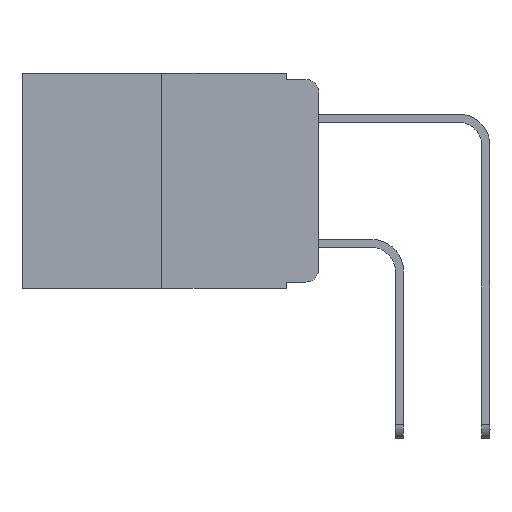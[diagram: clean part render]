
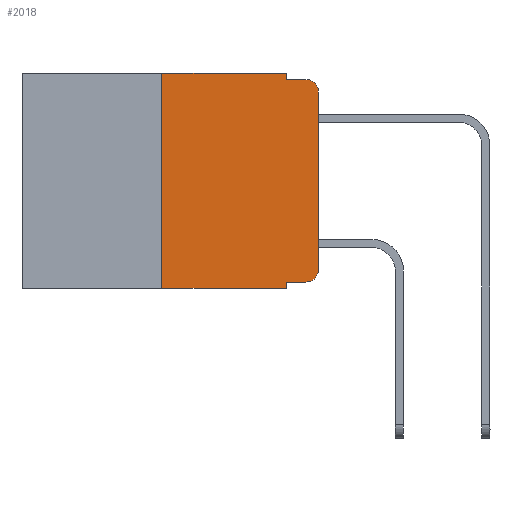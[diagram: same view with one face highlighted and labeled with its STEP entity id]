
A CAD part, left-side view. The second image highlights one B-rep face of the part: STEP entity #2018.
In plain terms, the highlighted planar face has unit normal (-1, 0, 0).
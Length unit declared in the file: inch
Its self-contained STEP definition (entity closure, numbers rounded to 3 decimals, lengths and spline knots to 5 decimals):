
#422 = EDGE_CURVE ( 'NONE', #14322, #1639, #7093, .T. ) ;
#611 = CARTESIAN_POINT ( 'NONE',  ( 0., 0.25, 0. ) ) ;
#840 = CARTESIAN_POINT ( 'NONE',  ( 0., 0.051, -0.333 ) ) ;
#1076 = EDGE_LOOP ( 'NONE', ( #9574, #23287, #19978, #2584, #23027, #23649, #20251, #6102, #7151, #8099 ) ) ;
#1297 = CARTESIAN_POINT ( 'NONE',  ( 0., 0.25, 0. ) ) ;
#1639 = VERTEX_POINT ( 'NONE', #19466 ) ;
#2018 = ADVANCED_FACE ( 'NONE', ( #4429 ), #2615, .F. ) ;
#2118 = CARTESIAN_POINT ( 'NONE',  ( 0., 0.051, 0. ) ) ;
#2147 = VERTEX_POINT ( 'NONE', #840 ) ;
#2360 = CARTESIAN_POINT ( 'NONE',  ( 0., 0.02, -0.03 ) ) ;
#2584 = ORIENTED_EDGE ( 'NONE', *, *, #422, .F. ) ;
#2593 = DIRECTION ( 'NONE',  ( 0., -1., 0. ) ) ;
#2615 = PLANE ( 'NONE',  #22516 ) ;
#2721 = DIRECTION ( 'NONE',  ( 0., 0., -1. ) ) ;
#2748 = VECTOR ( 'NONE', #12771, 39.37008 ) ;
#2932 = VECTOR ( 'NONE', #7549, 39.37008 ) ;
#3900 = DIRECTION ( 'NONE',  ( 0., -1., 0. ) ) ;
#3923 = EDGE_CURVE ( 'NONE', #11916, #7514, #4815, .T. ) ;
#4429 = FACE_OUTER_BOUND ( 'NONE', #1076, .T. ) ;
#4815 = LINE ( 'NONE', #10247, #19040 ) ;
#4859 = VECTOR ( 'NONE', #5276, 39.37008 ) ;
#4883 = VECTOR ( 'NONE', #5270, 39.37008 ) ;
#5023 = EDGE_CURVE ( 'NONE', #5339, #14322, #12719, .T. ) ;
#5270 = DIRECTION ( 'NONE',  ( 0., 0., 1. ) ) ;
#5276 = DIRECTION ( 'NONE',  ( 0., 0., 1. ) ) ;
#5339 = VERTEX_POINT ( 'NONE', #611 ) ;
#5505 = CARTESIAN_POINT ( 'NONE',  ( 0., 0.051, -0.343 ) ) ;
#6102 = ORIENTED_EDGE ( 'NONE', *, *, #18619, .F. ) ;
#6596 = DIRECTION ( 'NONE',  ( 1., 0., 0. ) ) ;
#6628 = EDGE_CURVE ( 'NONE', #2147, #13304, #19169, .T. ) ;
#7093 = LINE ( 'NONE', #19825, #2748 ) ;
#7151 = ORIENTED_EDGE ( 'NONE', *, *, #6628, .T. ) ;
#7514 = VERTEX_POINT ( 'NONE', #5505 ) ;
#7549 = DIRECTION ( 'NONE',  ( 0., 0., -1. ) ) ;
#8099 = ORIENTED_EDGE ( 'NONE', *, *, #9639, .T. ) ;
#8735 = CIRCLE ( 'NONE', #19583, 0.02 ) ;
#9193 = DIRECTION ( 'NONE',  ( 0., 0., -1. ) ) ;
#9363 = LINE ( 'NONE', #2118, #2932 ) ;
#9413 = VERTEX_POINT ( 'NONE', #15880 ) ;
#9574 = ORIENTED_EDGE ( 'NONE', *, *, #19260, .T. ) ;
#9639 = EDGE_CURVE ( 'NONE', #13304, #9413, #15652, .T. ) ;
#9912 = VECTOR ( 'NONE', #10658, 39.37008 ) ;
#9978 = CARTESIAN_POINT ( 'NONE',  ( 0., 0.473, 0. ) ) ;
#10247 = CARTESIAN_POINT ( 'NONE',  ( 0., 0.473, -0.343 ) ) ;
#10317 = VECTOR ( 'NONE', #2593, 39.37008 ) ;
#10330 = CARTESIAN_POINT ( 'NONE',  ( 0., 0.051, -0.333 ) ) ;
#10658 = DIRECTION ( 'NONE',  ( 0., -1., 0. ) ) ;
#11916 = VERTEX_POINT ( 'NONE', #13614 ) ;
#12398 = VERTEX_POINT ( 'NONE', #16133 ) ;
#12719 = LINE ( 'NONE', #23633, #9912 ) ;
#12734 = EDGE_CURVE ( 'NONE', #1639, #22343, #19135, .T. ) ;
#12771 = DIRECTION ( 'NONE',  ( 0., 0., -1. ) ) ;
#12829 = DIRECTION ( 'NONE',  ( -1., 0., 0. ) ) ;
#13304 = VERTEX_POINT ( 'NONE', #15470 ) ;
#13472 = DIRECTION ( 'NONE',  ( -1., 0., 0. ) ) ;
#13614 = CARTESIAN_POINT ( 'NONE',  ( 0., 0.25, -0.343 ) ) ;
#14322 = VERTEX_POINT ( 'NONE', #22145 ) ;
#14596 = LINE ( 'NONE', #1297, #4859 ) ;
#14657 = CARTESIAN_POINT ( 'NONE',  ( 0., 0.02, -0.313 ) ) ;
#15470 = CARTESIAN_POINT ( 'NONE',  ( 0., 0.02, -0.333 ) ) ;
#15652 = CIRCLE ( 'NONE', #23403, 0.02 ) ;
#15880 = CARTESIAN_POINT ( 'NONE',  ( 0., 0., -0.313 ) ) ;
#16133 = CARTESIAN_POINT ( 'NONE',  ( 0., 0., -0.03 ) ) ;
#17514 = DIRECTION ( 'NONE',  ( 0., -1., 0. ) ) ;
#18619 = EDGE_CURVE ( 'NONE', #2147, #7514, #9363, .T. ) ;
#19040 = VECTOR ( 'NONE', #17514, 39.37008 ) ;
#19135 = LINE ( 'NONE', #20461, #23629 ) ;
#19169 = LINE ( 'NONE', #10330, #10317 ) ;
#19260 = EDGE_CURVE ( 'NONE', #9413, #12398, #23201, .T. ) ;
#19297 = CARTESIAN_POINT ( 'NONE',  ( 0., 0.02, -0.01 ) ) ;
#19466 = CARTESIAN_POINT ( 'NONE',  ( 0., 0.051, -0.01 ) ) ;
#19583 = AXIS2_PLACEMENT_3D ( 'NONE', #2360, #13472, #2721 ) ;
#19825 = CARTESIAN_POINT ( 'NONE',  ( 0., 0.051, 0. ) ) ;
#19978 = ORIENTED_EDGE ( 'NONE', *, *, #12734, .F. ) ;
#20251 = ORIENTED_EDGE ( 'NONE', *, *, #3923, .T. ) ;
#20461 = CARTESIAN_POINT ( 'NONE',  ( 0., 0.051, -0.01 ) ) ;
#20703 = EDGE_CURVE ( 'NONE', #11916, #5339, #14596, .T. ) ;
#20955 = EDGE_CURVE ( 'NONE', #12398, #22343, #8735, .T. ) ;
#21109 = DIRECTION ( 'NONE',  ( 0., 0., -1. ) ) ;
#21725 = CARTESIAN_POINT ( 'NONE',  ( 0., 0., 0. ) ) ;
#22145 = CARTESIAN_POINT ( 'NONE',  ( 0., 0.051, 0. ) ) ;
#22343 = VERTEX_POINT ( 'NONE', #19297 ) ;
#22516 = AXIS2_PLACEMENT_3D ( 'NONE', #9978, #6596, #21109 ) ;
#23027 = ORIENTED_EDGE ( 'NONE', *, *, #5023, .F. ) ;
#23201 = LINE ( 'NONE', #21725, #4883 ) ;
#23287 = ORIENTED_EDGE ( 'NONE', *, *, #20955, .T. ) ;
#23403 = AXIS2_PLACEMENT_3D ( 'NONE', #14657, #12829, #9193 ) ;
#23629 = VECTOR ( 'NONE', #3900, 39.37008 ) ;
#23633 = CARTESIAN_POINT ( 'NONE',  ( 0., 0.473, 0. ) ) ;
#23649 = ORIENTED_EDGE ( 'NONE', *, *, #20703, .F. ) ;
